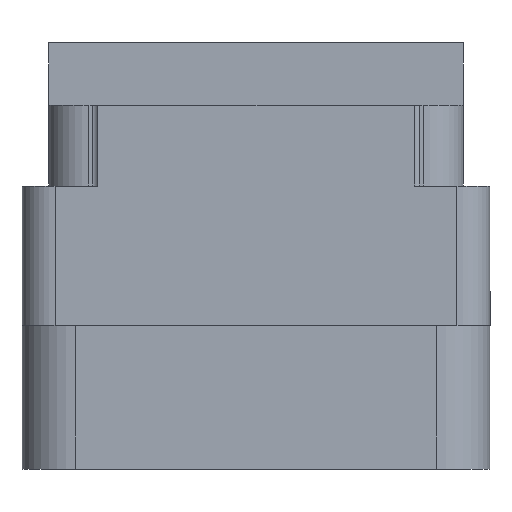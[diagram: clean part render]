
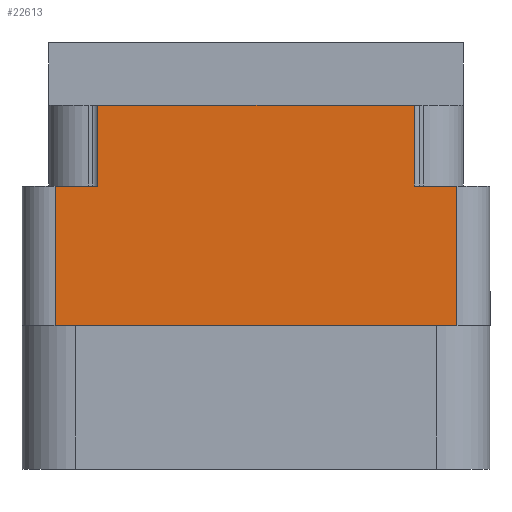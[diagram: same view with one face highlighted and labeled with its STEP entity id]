
A CAD part, left-side view. The second image highlights one B-rep face of the part: STEP entity #22613.
In plain terms, the highlighted planar face has unit normal (-1, 0, 0).
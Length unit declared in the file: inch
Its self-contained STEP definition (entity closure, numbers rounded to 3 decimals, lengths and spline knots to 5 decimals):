
#567 = CARTESIAN_POINT ( 'NONE',  ( -1., -0.296, -0.268 ) ) ;
#761 = DIRECTION ( 'NONE',  ( 0., -1., 0. ) ) ;
#859 = VERTEX_POINT ( 'NONE', #567 ) ;
#1368 = ORIENTED_EDGE ( 'NONE', *, *, #26086, .F. ) ;
#2714 = VERTEX_POINT ( 'NONE', #12686 ) ;
#2935 = AXIS2_PLACEMENT_3D ( 'NONE', #7979, #18961, #27911 ) ;
#3059 = CARTESIAN_POINT ( 'NONE',  ( -1., 0.376, -0.268 ) ) ;
#3406 = PLANE ( 'NONE',  #2935 ) ;
#3678 = DIRECTION ( 'NONE',  ( 0., 0., 1. ) ) ;
#3808 = CARTESIAN_POINT ( 'NONE',  ( -1., 0.376, -0.529 ) ) ;
#3890 = CARTESIAN_POINT ( 'NONE',  ( -1., 0.296, -0.117 ) ) ;
#4485 = CARTESIAN_POINT ( 'NONE',  ( -1., 0.438, -0.117 ) ) ;
#4836 = VECTOR ( 'NONE', #8899, 39.37008 ) ;
#5733 = CARTESIAN_POINT ( 'NONE',  ( -1., 0., -0.529 ) ) ;
#5928 = DIRECTION ( 'NONE',  ( 0., -1., 0. ) ) ;
#6321 = VERTEX_POINT ( 'NONE', #14289 ) ;
#6917 = LINE ( 'NONE', #14888, #21142 ) ;
#7442 = LINE ( 'NONE', #27581, #19262 ) ;
#7979 = CARTESIAN_POINT ( 'NONE',  ( -1., -0.376, -0.798 ) ) ;
#8578 = ORIENTED_EDGE ( 'NONE', *, *, #26430, .T. ) ;
#8721 = CARTESIAN_POINT ( 'NONE',  ( -1., 0.376, -0.798 ) ) ;
#8899 = DIRECTION ( 'NONE',  ( 0., 0., 1. ) ) ;
#10213 = CARTESIAN_POINT ( 'NONE',  ( -1., -0.376, -0.529 ) ) ;
#10324 = VECTOR ( 'NONE', #5928, 39.37008 ) ;
#10387 = DIRECTION ( 'NONE',  ( 0., 0., 1. ) ) ;
#11244 = EDGE_CURVE ( 'NONE', #6321, #15662, #6917, .T. ) ;
#11528 = ORIENTED_EDGE ( 'NONE', *, *, #23080, .F. ) ;
#12009 = EDGE_CURVE ( 'NONE', #16972, #28537, #21152, .T. ) ;
#12686 = CARTESIAN_POINT ( 'NONE',  ( -1., -0.376, -0.268 ) ) ;
#12999 = LINE ( 'NONE', #24445, #13357 ) ;
#13051 = DIRECTION ( 'NONE',  ( 0., -1., 0. ) ) ;
#13327 = ORIENTED_EDGE ( 'NONE', *, *, #22349, .F. ) ;
#13357 = VECTOR ( 'NONE', #17935, 39.37008 ) ;
#14289 = CARTESIAN_POINT ( 'NONE',  ( -1., 0.296, -0.268 ) ) ;
#14378 = ORIENTED_EDGE ( 'NONE', *, *, #14841, .T. ) ;
#14591 = ORIENTED_EDGE ( 'NONE', *, *, #24144, .T. ) ;
#14841 = EDGE_CURVE ( 'NONE', #25824, #2714, #12999, .T. ) ;
#14888 = CARTESIAN_POINT ( 'NONE',  ( -1., 0.296, -0.268 ) ) ;
#14945 = LINE ( 'NONE', #22146, #25957 ) ;
#15662 = VERTEX_POINT ( 'NONE', #3890 ) ;
#15900 = VERTEX_POINT ( 'NONE', #16847 ) ;
#15908 = EDGE_LOOP ( 'NONE', ( #25174, #8578, #14378, #1368, #14591, #13327, #28490, #11528 ) ) ;
#16847 = CARTESIAN_POINT ( 'NONE',  ( -1., -0.296, -0.117 ) ) ;
#16972 = VERTEX_POINT ( 'NONE', #3808 ) ;
#17935 = DIRECTION ( 'NONE',  ( 0., 0., 1. ) ) ;
#18961 = DIRECTION ( 'NONE',  ( -1., 0., 0. ) ) ;
#19262 = VECTOR ( 'NONE', #761, 39.37008 ) ;
#20925 = LINE ( 'NONE', #21370, #27830 ) ;
#21142 = VECTOR ( 'NONE', #3678, 39.37008 ) ;
#21152 = LINE ( 'NONE', #8721, #4836 ) ;
#21329 = LINE ( 'NONE', #4485, #24394 ) ;
#21370 = CARTESIAN_POINT ( 'NONE',  ( -1., -0.296, -0.268 ) ) ;
#22146 = CARTESIAN_POINT ( 'NONE',  ( -1., -0.296, -0.268 ) ) ;
#22349 = EDGE_CURVE ( 'NONE', #15662, #15900, #21329, .T. ) ;
#22613 = ADVANCED_FACE ( 'NONE', ( #23720 ), #3406, .T. ) ;
#23080 = EDGE_CURVE ( 'NONE', #28537, #6321, #7442, .T. ) ;
#23720 = FACE_OUTER_BOUND ( 'NONE', #15908, .T. ) ;
#24144 = EDGE_CURVE ( 'NONE', #859, #15900, #20925, .T. ) ;
#24394 = VECTOR ( 'NONE', #26554, 39.37008 ) ;
#24445 = CARTESIAN_POINT ( 'NONE',  ( -1., -0.376, -0.798 ) ) ;
#25174 = ORIENTED_EDGE ( 'NONE', *, *, #12009, .F. ) ;
#25824 = VERTEX_POINT ( 'NONE', #10213 ) ;
#25957 = VECTOR ( 'NONE', #13051, 39.37008 ) ;
#26086 = EDGE_CURVE ( 'NONE', #859, #2714, #14945, .T. ) ;
#26430 = EDGE_CURVE ( 'NONE', #16972, #25824, #28682, .T. ) ;
#26554 = DIRECTION ( 'NONE',  ( 0., -1., 0. ) ) ;
#27581 = CARTESIAN_POINT ( 'NONE',  ( -1., 0.438, -0.268 ) ) ;
#27830 = VECTOR ( 'NONE', #10387, 39.37008 ) ;
#27911 = DIRECTION ( 'NONE',  ( 0., 0., 1. ) ) ;
#28490 = ORIENTED_EDGE ( 'NONE', *, *, #11244, .F. ) ;
#28537 = VERTEX_POINT ( 'NONE', #3059 ) ;
#28682 = LINE ( 'NONE', #5733, #10324 ) ;
